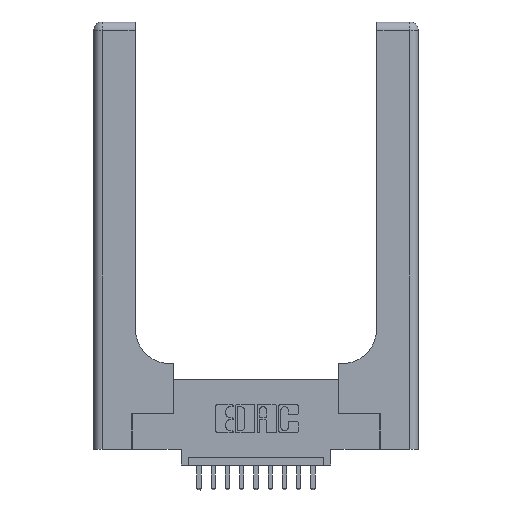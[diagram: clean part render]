
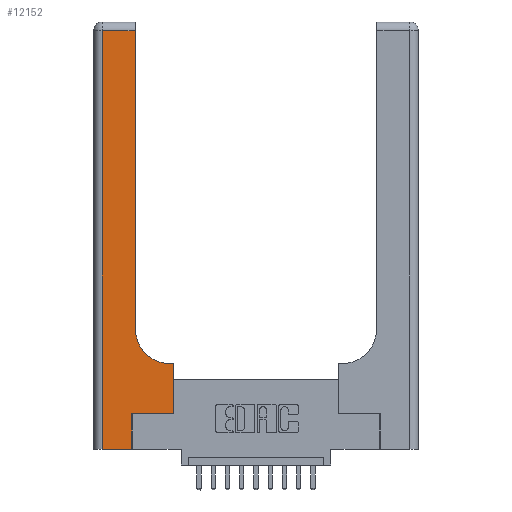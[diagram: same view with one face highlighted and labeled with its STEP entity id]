
A CAD part, top view. The second image highlights one B-rep face of the part: STEP entity #12152.
In plain terms, the highlighted planar face has unit normal (0, 0, 1).
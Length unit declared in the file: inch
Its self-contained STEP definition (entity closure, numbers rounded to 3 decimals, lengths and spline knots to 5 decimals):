
#101 = EDGE_CURVE ( 'NONE', #4835, #12401, #9275, .T. ) ;
#169 = CARTESIAN_POINT ( 'NONE',  ( 0.06, 2.94, 0.37 ) ) ;
#281 = CARTESIAN_POINT ( 'NONE',  ( 0., 0., 0.37 ) ) ;
#632 = CARTESIAN_POINT ( 'NONE',  ( 0.06, 0., 0.37 ) ) ;
#692 = LINE ( 'NONE', #1014, #15181 ) ;
#1014 = CARTESIAN_POINT ( 'NONE',  ( 0., 2.94, 0.37 ) ) ;
#1015 = AXIS2_PLACEMENT_3D ( 'NONE', #8484, #13475, #9671 ) ;
#1017 = VECTOR ( 'NONE', #14166, 39.37008 ) ;
#1383 = ORIENTED_EDGE ( 'NONE', *, *, #101, .T. ) ;
#1535 = CARTESIAN_POINT ( 'NONE',  ( 0.5585, 0.6, 0.37 ) ) ;
#1771 = VERTEX_POINT ( 'NONE', #1535 ) ;
#1853 = LINE ( 'NONE', #2536, #15160 ) ;
#2303 = ORIENTED_EDGE ( 'NONE', *, *, #8215, .T. ) ;
#2359 = VECTOR ( 'NONE', #13710, 39.37008 ) ;
#2469 = LINE ( 'NONE', #2705, #12103 ) ;
#2536 = CARTESIAN_POINT ( 'NONE',  ( 0.5585, 0.25, 0.37 ) ) ;
#2603 = CARTESIAN_POINT ( 'NONE',  ( 0.5585, 0.25, 0.37 ) ) ;
#2705 = CARTESIAN_POINT ( 'NONE',  ( 0.2915, 0.6, 0.37 ) ) ;
#2819 = DIRECTION ( 'NONE',  ( 1., 0., 0. ) ) ;
#3914 = ORIENTED_EDGE ( 'NONE', *, *, #6790, .T. ) ;
#4332 = ORIENTED_EDGE ( 'NONE', *, *, #8988, .T. ) ;
#4379 = VECTOR ( 'NONE', #6255, 39.37008 ) ;
#4460 = PLANE ( 'NONE',  #1015 ) ;
#4549 = ORIENTED_EDGE ( 'NONE', *, *, #8604, .T. ) ;
#4598 = FACE_OUTER_BOUND ( 'NONE', #5467, .T. ) ;
#4835 = VERTEX_POINT ( 'NONE', #6930 ) ;
#5467 = EDGE_LOOP ( 'NONE', ( #10503, #4549, #15239, #7107, #3914, #1383, #4332, #10114, #2303 ) ) ;
#5849 = VECTOR ( 'NONE', #11412, 39.37008 ) ;
#6255 = DIRECTION ( 'NONE',  ( 0., -1., 0. ) ) ;
#6285 = DIRECTION ( 'NONE',  ( 1., 0., 0. ) ) ;
#6502 = DIRECTION ( 'NONE',  ( 0., 1., 0. ) ) ;
#6790 = EDGE_CURVE ( 'NONE', #8355, #4835, #14452, .T. ) ;
#6930 = CARTESIAN_POINT ( 'NONE',  ( 0.269, 0.25, 0.37 ) ) ;
#7107 = ORIENTED_EDGE ( 'NONE', *, *, #13151, .T. ) ;
#8215 = EDGE_CURVE ( 'NONE', #14368, #8353, #8702, .T. ) ;
#8353 = VERTEX_POINT ( 'NONE', #9608 ) ;
#8355 = VERTEX_POINT ( 'NONE', #16132 ) ;
#8484 = CARTESIAN_POINT ( 'NONE',  ( 0., 3., 0.37 ) ) ;
#8604 = EDGE_CURVE ( 'NONE', #15591, #14773, #692, .T. ) ;
#8615 = LINE ( 'NONE', #14347, #1017 ) ;
#8702 = CIRCLE ( 'NONE', #14976, 0.25 ) ;
#8783 = DIRECTION ( 'NONE',  ( 0., 0., -1. ) ) ;
#8988 = EDGE_CURVE ( 'NONE', #12401, #1771, #1853, .T. ) ;
#9275 = LINE ( 'NONE', #10120, #5849 ) ;
#9608 = CARTESIAN_POINT ( 'NONE',  ( 0.2915, 0.85, 0.37 ) ) ;
#9626 = CARTESIAN_POINT ( 'NONE',  ( 0.269, 0., 0.37 ) ) ;
#9671 = DIRECTION ( 'NONE',  ( -1., 0., 0. ) ) ;
#9974 = DIRECTION ( 'NONE',  ( -1., 0., 0. ) ) ;
#10114 = ORIENTED_EDGE ( 'NONE', *, *, #15814, .T. ) ;
#10120 = CARTESIAN_POINT ( 'NONE',  ( 0.269, 0.25, 0.37 ) ) ;
#10177 = CARTESIAN_POINT ( 'NONE',  ( 0.2915, 2.94, 0.37 ) ) ;
#10460 = DIRECTION ( 'NONE',  ( -1., 0., 0. ) ) ;
#10503 = ORIENTED_EDGE ( 'NONE', *, *, #10982, .T. ) ;
#10982 = EDGE_CURVE ( 'NONE', #8353, #15591, #8615, .T. ) ;
#11412 = DIRECTION ( 'NONE',  ( 1., 0., 0. ) ) ;
#11735 = CARTESIAN_POINT ( 'NONE',  ( 0.5415, 0.6, 0.37 ) ) ;
#12103 = VECTOR ( 'NONE', #10460, 39.37008 ) ;
#12152 = ADVANCED_FACE ( 'NONE', ( #4598 ), #4460, .F. ) ;
#12218 = VECTOR ( 'NONE', #2819, 39.37008 ) ;
#12401 = VERTEX_POINT ( 'NONE', #2603 ) ;
#12812 = EDGE_CURVE ( 'NONE', #14773, #16550, #14271, .T. ) ;
#13151 = EDGE_CURVE ( 'NONE', #16550, #8355, #15676, .T. ) ;
#13475 = DIRECTION ( 'NONE',  ( 0., 0., -1. ) ) ;
#13710 = DIRECTION ( 'NONE',  ( 0., 1., 0. ) ) ;
#14052 = CARTESIAN_POINT ( 'NONE',  ( 0.5415, 0.85, 0.37 ) ) ;
#14166 = DIRECTION ( 'NONE',  ( 0., 1., 0. ) ) ;
#14271 = LINE ( 'NONE', #16486, #4379 ) ;
#14347 = CARTESIAN_POINT ( 'NONE',  ( 0.2915, 3., 0.37 ) ) ;
#14368 = VERTEX_POINT ( 'NONE', #11735 ) ;
#14452 = LINE ( 'NONE', #9626, #2359 ) ;
#14773 = VERTEX_POINT ( 'NONE', #169 ) ;
#14976 = AXIS2_PLACEMENT_3D ( 'NONE', #14052, #8783, #6285 ) ;
#15160 = VECTOR ( 'NONE', #6502, 39.37008 ) ;
#15181 = VECTOR ( 'NONE', #9974, 39.37008 ) ;
#15239 = ORIENTED_EDGE ( 'NONE', *, *, #12812, .T. ) ;
#15591 = VERTEX_POINT ( 'NONE', #10177 ) ;
#15676 = LINE ( 'NONE', #281, #12218 ) ;
#15814 = EDGE_CURVE ( 'NONE', #1771, #14368, #2469, .T. ) ;
#16132 = CARTESIAN_POINT ( 'NONE',  ( 0.269, 0., 0.37 ) ) ;
#16486 = CARTESIAN_POINT ( 'NONE',  ( 0.06, 3., 0.37 ) ) ;
#16550 = VERTEX_POINT ( 'NONE', #632 ) ;
